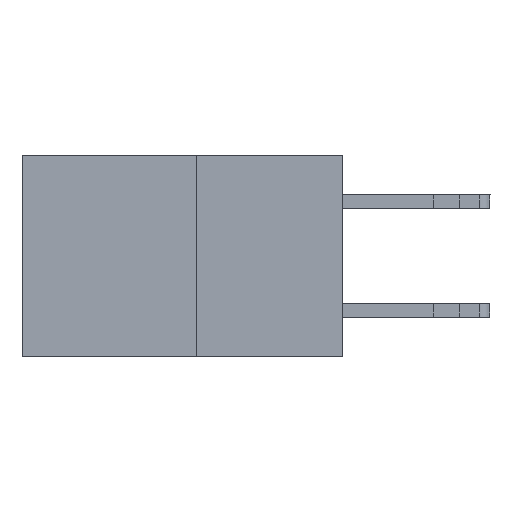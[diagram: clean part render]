
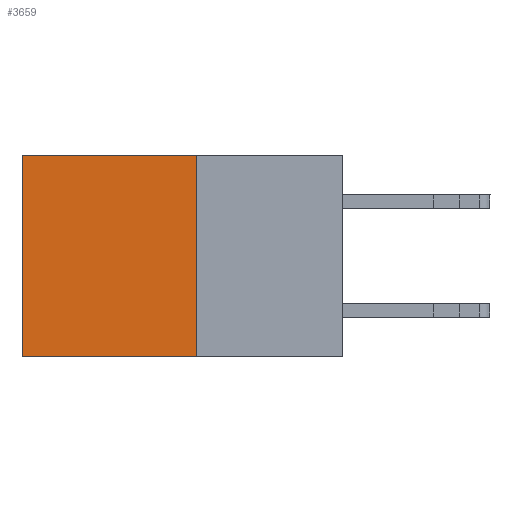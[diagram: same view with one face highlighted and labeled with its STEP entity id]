
A CAD part, left-side view. The second image highlights one B-rep face of the part: STEP entity #3659.
In plain terms, the highlighted planar face has unit normal (-1, 0, 0).
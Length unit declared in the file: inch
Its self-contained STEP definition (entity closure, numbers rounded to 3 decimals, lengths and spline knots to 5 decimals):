
#976 = VERTEX_POINT ( 'NONE', #14885 ) ;
#1065 = LINE ( 'NONE', #5144, #4398 ) ;
#1334 = CARTESIAN_POINT ( 'NONE',  ( 0.277, 0.27, 0. ) ) ;
#1350 = LINE ( 'NONE', #4107, #10328 ) ;
#1816 = FACE_OUTER_BOUND ( 'NONE', #5897, .T. ) ;
#3467 = VERTEX_POINT ( 'NONE', #6268 ) ;
#3659 = ADVANCED_FACE ( 'NONE', ( #1816 ), #6058, .F. ) ;
#3852 = EDGE_CURVE ( 'NONE', #14447, #11427, #8181, .T. ) ;
#4107 = CARTESIAN_POINT ( 'NONE',  ( 0.277, 0.27, -0.37 ) ) ;
#4398 = VECTOR ( 'NONE', #6436, 39.37008 ) ;
#4525 = AXIS2_PLACEMENT_3D ( 'NONE', #11702, #10324, #11967 ) ;
#4751 = VECTOR ( 'NONE', #11049, 39.37008 ) ;
#5144 = CARTESIAN_POINT ( 'NONE',  ( 0.277, 0.59, -0.37 ) ) ;
#5539 = ORIENTED_EDGE ( 'NONE', *, *, #6274, .T. ) ;
#5897 = EDGE_LOOP ( 'NONE', ( #5539, #10672, #7869, #11230 ) ) ;
#6058 = PLANE ( 'NONE',  #4525 ) ;
#6268 = CARTESIAN_POINT ( 'NONE',  ( 0.277, 0.27, -0.37 ) ) ;
#6274 = EDGE_CURVE ( 'NONE', #11427, #976, #1065, .T. ) ;
#6436 = DIRECTION ( 'NONE',  ( 0., 0., -1. ) ) ;
#6624 = CARTESIAN_POINT ( 'NONE',  ( 0.277, 0.27, -0.37 ) ) ;
#6821 = EDGE_CURVE ( 'NONE', #14447, #3467, #1350, .T. ) ;
#7839 = DIRECTION ( 'NONE',  ( 0., 1., 0. ) ) ;
#7869 = ORIENTED_EDGE ( 'NONE', *, *, #6821, .F. ) ;
#8181 = LINE ( 'NONE', #1334, #4751 ) ;
#10324 = DIRECTION ( 'NONE',  ( 1., 0., 0. ) ) ;
#10328 = VECTOR ( 'NONE', #12796, 39.37008 ) ;
#10672 = ORIENTED_EDGE ( 'NONE', *, *, #13805, .F. ) ;
#11049 = DIRECTION ( 'NONE',  ( 0., 1., 0. ) ) ;
#11230 = ORIENTED_EDGE ( 'NONE', *, *, #3852, .T. ) ;
#11427 = VERTEX_POINT ( 'NONE', #16465 ) ;
#11702 = CARTESIAN_POINT ( 'NONE',  ( 0.277, 0.27, -0.37 ) ) ;
#11967 = DIRECTION ( 'NONE',  ( 0., 0., -1. ) ) ;
#12796 = DIRECTION ( 'NONE',  ( 0., 0., -1. ) ) ;
#13805 = EDGE_CURVE ( 'NONE', #3467, #976, #14937, .T. ) ;
#14447 = VERTEX_POINT ( 'NONE', #17109 ) ;
#14885 = CARTESIAN_POINT ( 'NONE',  ( 0.277, 0.59, -0.37 ) ) ;
#14937 = LINE ( 'NONE', #6624, #16461 ) ;
#16461 = VECTOR ( 'NONE', #7839, 39.37008 ) ;
#16465 = CARTESIAN_POINT ( 'NONE',  ( 0.277, 0.59, 0. ) ) ;
#17109 = CARTESIAN_POINT ( 'NONE',  ( 0.277, 0.27, 0. ) ) ;
